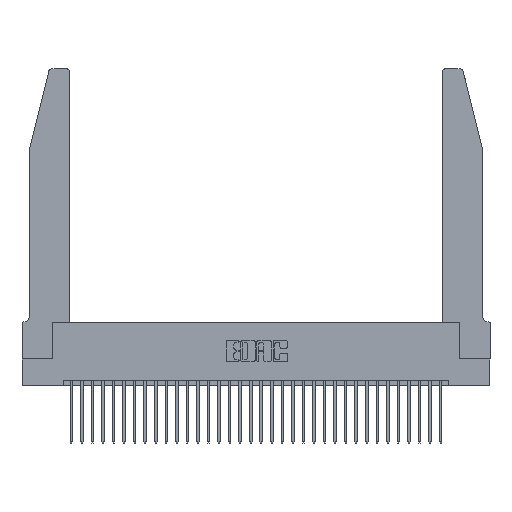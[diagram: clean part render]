
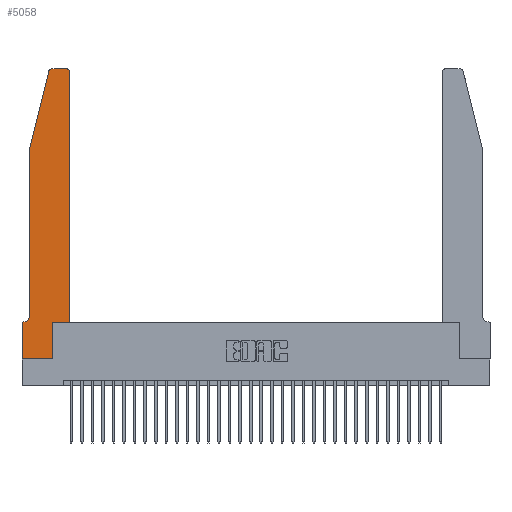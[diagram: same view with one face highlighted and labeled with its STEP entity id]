
A CAD part, top view. The second image highlights one B-rep face of the part: STEP entity #5058.
In plain terms, the highlighted planar face has unit normal (0, 0, 1).
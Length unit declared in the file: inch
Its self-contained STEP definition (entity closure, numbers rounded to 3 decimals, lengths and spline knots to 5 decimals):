
#1 = DIRECTION ( 'NONE',  ( 0., 1., 0. ) ) ;
#185 = CARTESIAN_POINT ( 'NONE',  ( 0., 0.35, 0.37 ) ) ;
#429 = CARTESIAN_POINT ( 'NONE',  ( 0.0055, 0.42, 0.37 ) ) ;
#523 = CARTESIAN_POINT ( 'NONE',  ( 0.0055, 0.35, 0.37 ) ) ;
#572 = DIRECTION ( 'NONE',  ( 0., -1., 0. ) ) ;
#1466 = ORIENTED_EDGE ( 'NONE', *, *, #17574, .T. ) ;
#1498 = VERTEX_POINT ( 'NONE', #523 ) ;
#1677 = VECTOR ( 'NONE', #2412, 39.37008 ) ;
#2344 = VERTEX_POINT ( 'NONE', #19566 ) ;
#2412 = DIRECTION ( 'NONE',  ( 1., 0., 0. ) ) ;
#2486 = LINE ( 'NONE', #28660, #1677 ) ;
#2883 = EDGE_CURVE ( 'NONE', #1498, #28347, #4114, .T. ) ;
#3044 = DIRECTION ( 'NONE',  ( -1., 0., 0. ) ) ;
#3376 = VECTOR ( 'NONE', #572, 39.37008 ) ;
#3687 = ORIENTED_EDGE ( 'NONE', *, *, #30821, .T. ) ;
#3985 = DIRECTION ( 'NONE',  ( 0., -1., 0. ) ) ;
#4114 = LINE ( 'NONE', #16801, #10356 ) ;
#4447 = VERTEX_POINT ( 'NONE', #17616 ) ;
#4925 = VERTEX_POINT ( 'NONE', #14452 ) ;
#4977 = DIRECTION ( 'NONE',  ( 0., 0., 1. ) ) ;
#5058 = ADVANCED_FACE ( 'NONE', ( #13466 ), #12395, .T. ) ;
#5081 = CARTESIAN_POINT ( 'NONE',  ( 0.4505, 0.35, 0.37 ) ) ;
#6385 = CARTESIAN_POINT ( 'NONE',  ( 0., 0., 0.37 ) ) ;
#6880 = VERTEX_POINT ( 'NONE', #6385 ) ;
#7069 = ORIENTED_EDGE ( 'NONE', *, *, #22116, .T. ) ;
#7211 = ORIENTED_EDGE ( 'NONE', *, *, #2883, .T. ) ;
#7382 = VECTOR ( 'NONE', #31055, 39.37008 ) ;
#7500 = VECTOR ( 'NONE', #1, 39.37008 ) ;
#8259 = VECTOR ( 'NONE', #24168, 39.37008 ) ;
#9630 = LINE ( 'NONE', #17159, #10464 ) ;
#10356 = VECTOR ( 'NONE', #19432, 39.37008 ) ;
#10464 = VECTOR ( 'NONE', #3985, 39.37008 ) ;
#10575 = ORIENTED_EDGE ( 'NONE', *, *, #20160, .T. ) ;
#11112 = EDGE_CURVE ( 'NONE', #29727, #4925, #21486, .T. ) ;
#12144 = CARTESIAN_POINT ( 'NONE',  ( 0.0755, 0.42, 0.37 ) ) ;
#12395 = PLANE ( 'NONE',  #25360 ) ;
#12834 = ORIENTED_EDGE ( 'NONE', *, *, #26912, .T. ) ;
#13466 = FACE_OUTER_BOUND ( 'NONE', #14661, .T. ) ;
#13467 = VERTEX_POINT ( 'NONE', #28998 ) ;
#13475 = CIRCLE ( 'NONE', #22386, 0.07 ) ;
#13687 = CARTESIAN_POINT ( 'NONE',  ( 0., 0., 0.37 ) ) ;
#13789 = CARTESIAN_POINT ( 'NONE',  ( 0.2865, 0., 0.37 ) ) ;
#14031 = CIRCLE ( 'NONE', #18845, 0.03 ) ;
#14450 = CARTESIAN_POINT ( 'NONE',  ( 0.284, 2.72, 0.37 ) ) ;
#14452 = CARTESIAN_POINT ( 'NONE',  ( 0.2865, 0.35, 0.37 ) ) ;
#14661 = EDGE_LOOP ( 'NONE', ( #17512, #22267, #27879, #12834, #19263, #7211, #1466, #10575, #19935, #3687, #7069, #15186 ) ) ;
#14668 = DIRECTION ( 'NONE',  ( 1., 0., 0. ) ) ;
#14908 = CARTESIAN_POINT ( 'NONE',  ( 0.4505, 2.72, 0.37 ) ) ;
#15186 = ORIENTED_EDGE ( 'NONE', *, *, #30186, .T. ) ;
#16801 = CARTESIAN_POINT ( 'NONE',  ( 0.0755, 0.35, 0.37 ) ) ;
#17115 = DIRECTION ( 'NONE',  ( 1., 0., 0. ) ) ;
#17159 = CARTESIAN_POINT ( 'NONE',  ( 0.0755, 2., 0.37 ) ) ;
#17512 = ORIENTED_EDGE ( 'NONE', *, *, #22568, .T. ) ;
#17574 = EDGE_CURVE ( 'NONE', #28347, #6880, #22709, .T. ) ;
#17616 = CARTESIAN_POINT ( 'NONE',  ( 0.4205, 2.75, 0.37 ) ) ;
#17643 = LINE ( 'NONE', #32873, #18470 ) ;
#17681 = DIRECTION ( 'NONE',  ( 1., 0., 0. ) ) ;
#18419 = CARTESIAN_POINT ( 'NONE',  ( 0.2865, 0.35, 0.37 ) ) ;
#18470 = VECTOR ( 'NONE', #14668, 39.37008 ) ;
#18837 = DIRECTION ( 'NONE',  ( 0., 0., -1. ) ) ;
#18845 = AXIS2_PLACEMENT_3D ( 'NONE', #20759, #4977, #23391 ) ;
#19045 = VERTEX_POINT ( 'NONE', #28327 ) ;
#19263 = ORIENTED_EDGE ( 'NONE', *, *, #32952, .T. ) ;
#19432 = DIRECTION ( 'NONE',  ( -1., 0., 0. ) ) ;
#19566 = CARTESIAN_POINT ( 'NONE',  ( 0.25487, 2.72718, 0.37 ) ) ;
#19935 = ORIENTED_EDGE ( 'NONE', *, *, #11112, .T. ) ;
#20109 = EDGE_CURVE ( 'NONE', #19045, #2344, #20919, .T. ) ;
#20160 = EDGE_CURVE ( 'NONE', #6880, #29727, #17643, .T. ) ;
#20759 = CARTESIAN_POINT ( 'NONE',  ( 0.4205, 2.72, 0.37 ) ) ;
#20919 = CIRCLE ( 'NONE', #27615, 0.03 ) ;
#21486 = LINE ( 'NONE', #18419, #7500 ) ;
#22116 = EDGE_CURVE ( 'NONE', #31570, #30361, #23040, .T. ) ;
#22183 = LINE ( 'NONE', #28455, #7382 ) ;
#22267 = ORIENTED_EDGE ( 'NONE', *, *, #20109, .T. ) ;
#22386 = AXIS2_PLACEMENT_3D ( 'NONE', #429, #18837, #3044 ) ;
#22568 = EDGE_CURVE ( 'NONE', #4447, #19045, #22183, .T. ) ;
#22709 = LINE ( 'NONE', #13687, #3376 ) ;
#22802 = CARTESIAN_POINT ( 'NONE',  ( 0., 0.35, 0.37 ) ) ;
#23040 = LINE ( 'NONE', #26803, #8259 ) ;
#23240 = DIRECTION ( 'NONE',  ( -0.239, -0.971, 0. ) ) ;
#23348 = CARTESIAN_POINT ( 'NONE',  ( 0.0755, 2., 0.37 ) ) ;
#23391 = DIRECTION ( 'NONE',  ( 1., 0., 0. ) ) ;
#23477 = VECTOR ( 'NONE', #23240, 39.37008 ) ;
#24168 = DIRECTION ( 'NONE',  ( 0., 1., 0. ) ) ;
#24273 = LINE ( 'NONE', #23348, #23477 ) ;
#25360 = AXIS2_PLACEMENT_3D ( 'NONE', #22802, #33207, #17681 ) ;
#26803 = CARTESIAN_POINT ( 'NONE',  ( 0.4505, 0.35, 0.37 ) ) ;
#26912 = EDGE_CURVE ( 'NONE', #13467, #33759, #9630, .T. ) ;
#27615 = AXIS2_PLACEMENT_3D ( 'NONE', #14450, #32651, #17115 ) ;
#27879 = ORIENTED_EDGE ( 'NONE', *, *, #30799, .T. ) ;
#28327 = CARTESIAN_POINT ( 'NONE',  ( 0.284, 2.75, 0.37 ) ) ;
#28347 = VERTEX_POINT ( 'NONE', #185 ) ;
#28455 = CARTESIAN_POINT ( 'NONE',  ( 0.2605, 2.75, 0.37 ) ) ;
#28660 = CARTESIAN_POINT ( 'NONE',  ( 0.4505, 0.35, 0.37 ) ) ;
#28998 = CARTESIAN_POINT ( 'NONE',  ( 0.0755, 2., 0.37 ) ) ;
#29727 = VERTEX_POINT ( 'NONE', #13789 ) ;
#30186 = EDGE_CURVE ( 'NONE', #30361, #4447, #14031, .T. ) ;
#30361 = VERTEX_POINT ( 'NONE', #14908 ) ;
#30799 = EDGE_CURVE ( 'NONE', #2344, #13467, #24273, .T. ) ;
#30821 = EDGE_CURVE ( 'NONE', #4925, #31570, #2486, .T. ) ;
#31055 = DIRECTION ( 'NONE',  ( -1., 0., 0. ) ) ;
#31570 = VERTEX_POINT ( 'NONE', #5081 ) ;
#32651 = DIRECTION ( 'NONE',  ( 0., 0., 1. ) ) ;
#32873 = CARTESIAN_POINT ( 'NONE',  ( 0., 0., 0.37 ) ) ;
#32952 = EDGE_CURVE ( 'NONE', #33759, #1498, #13475, .T. ) ;
#33207 = DIRECTION ( 'NONE',  ( 0., 0., 1. ) ) ;
#33759 = VERTEX_POINT ( 'NONE', #12144 ) ;
